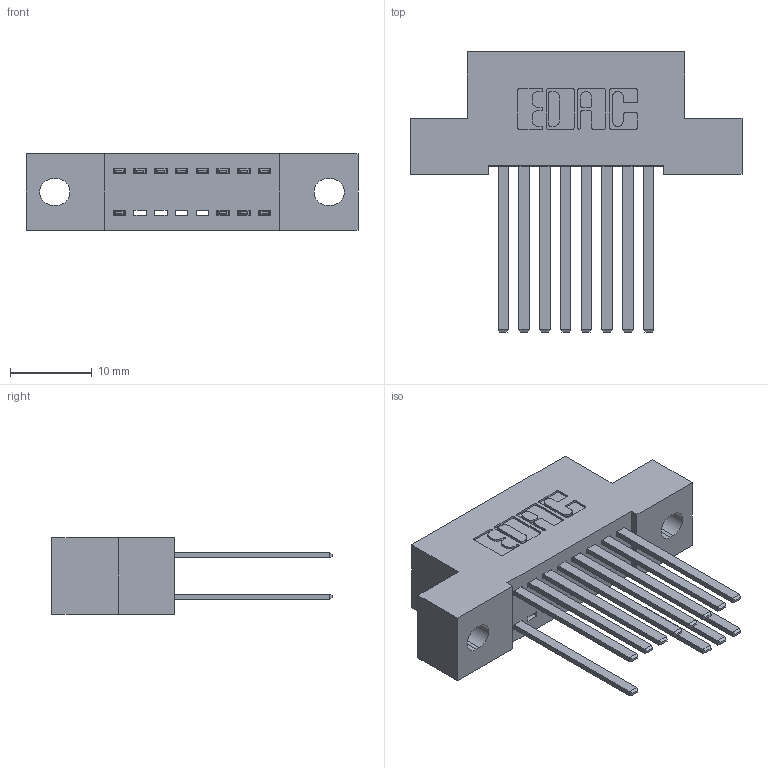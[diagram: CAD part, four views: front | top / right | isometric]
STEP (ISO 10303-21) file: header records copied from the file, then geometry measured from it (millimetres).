
FILE_DESCRIPTION (( 'STEP AP203' ), '1' );
FILE_NAME ('392-016-544-202.STEP', '2018-08-15T02:17:59', ( '' ), ( '' ), 'SwSTEP 2.0', 'SolidWorks 2016', '' );
FILE_SCHEMA (( 'CONFIG_CONTROL_DESIGN' ));
Length unit declared in the file: inch
Products named in the file (3): 392-016-544-202; 342 Part_.128 Slot; 345-292-001_345-293-144
Assembly tree (13 placements, depth 2):
  392-016-544-202
    342 Part_.128 Slot
    345-292-001_345-293-144  x12
Bounding box: 40.64 x 34.3 x 9.4 mm (x, y, z)
Volume: 3570.6 mm3; surface area: 5000.7 mm2
Topology: 13 solids, 13 shells, 690 faces, 2039 edges, 1342 vertices
Faces by surface type: plane 478, cylinder 212
Entity records: 9235 total; most frequent: CARTESIAN_POINT 1586, ORIENTED_EDGE 1526, DIRECTION 1407, EDGE_CURVE 763, VECTOR 639, LINE 639, VERTEX_POINT 506, AXIS2_PLACEMENT_3D 384
